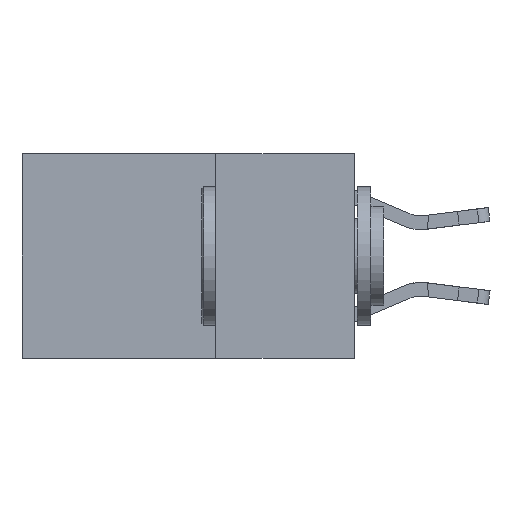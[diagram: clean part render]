
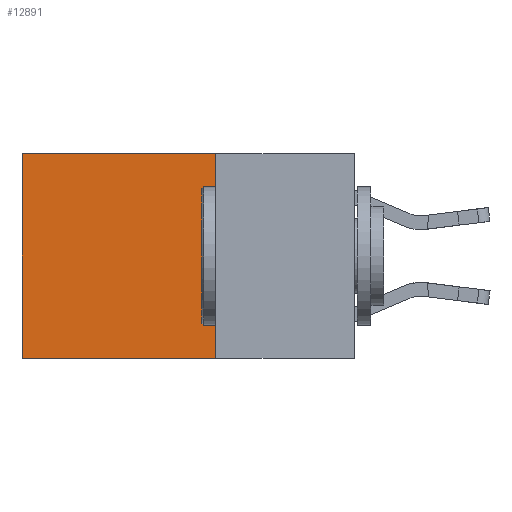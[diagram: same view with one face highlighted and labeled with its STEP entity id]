
A CAD part, left-side view. The second image highlights one B-rep face of the part: STEP entity #12891.
In plain terms, the highlighted planar face has unit normal (-1, 0, 0).
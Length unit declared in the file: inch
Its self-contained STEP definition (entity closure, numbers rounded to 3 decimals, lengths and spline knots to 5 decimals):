
#623 = AXIS2_PLACEMENT_3D ( 'NONE', #16962, #15904, #2747 ) ;
#1274 = VERTEX_POINT ( 'NONE', #6237 ) ;
#1574 = CARTESIAN_POINT ( 'NONE',  ( 0.2625, 0.25, 0. ) ) ;
#2537 = LINE ( 'NONE', #6964, #4032 ) ;
#2646 = PLANE ( 'NONE',  #623 ) ;
#2747 = DIRECTION ( 'NONE',  ( 0., 0., -1. ) ) ;
#2769 = ORIENTED_EDGE ( 'NONE', *, *, #17958, .F. ) ;
#3124 = VERTEX_POINT ( 'NONE', #14053 ) ;
#3986 = FACE_OUTER_BOUND ( 'NONE', #12010, .T. ) ;
#4032 = VECTOR ( 'NONE', #13962, 39.37008 ) ;
#6237 = CARTESIAN_POINT ( 'NONE',  ( 0.2625, 0.6, -0.37 ) ) ;
#6335 = EDGE_CURVE ( 'NONE', #3124, #1274, #2537, .T. ) ;
#6521 = DIRECTION ( 'NONE',  ( 0., 0., -1. ) ) ;
#6964 = CARTESIAN_POINT ( 'NONE',  ( 0.2625, 0.6, 0. ) ) ;
#7256 = DIRECTION ( 'NONE',  ( 0., 1., 0. ) ) ;
#7347 = LINE ( 'NONE', #1574, #14202 ) ;
#8284 = ORIENTED_EDGE ( 'NONE', *, *, #6335, .T. ) ;
#8939 = EDGE_CURVE ( 'NONE', #15135, #14184, #18432, .T. ) ;
#9906 = CARTESIAN_POINT ( 'NONE',  ( 0.2625, 0.25, 0. ) ) ;
#10504 = LINE ( 'NONE', #13473, #16674 ) ;
#11165 = VECTOR ( 'NONE', #6521, 39.37008 ) ;
#12010 = EDGE_LOOP ( 'NONE', ( #8284, #2769, #17851, #18306 ) ) ;
#12643 = CARTESIAN_POINT ( 'NONE',  ( 0.2625, 0.25, 0. ) ) ;
#12649 = CARTESIAN_POINT ( 'NONE',  ( 0.2625, 0.25, -0.37 ) ) ;
#12891 = ADVANCED_FACE ( 'NONE', ( #3986 ), #2646, .F. ) ;
#13473 = CARTESIAN_POINT ( 'NONE',  ( 0.2625, 0.25, -0.37 ) ) ;
#13962 = DIRECTION ( 'NONE',  ( 0., 0., -1. ) ) ;
#14053 = CARTESIAN_POINT ( 'NONE',  ( 0.2625, 0.6, 0. ) ) ;
#14184 = VERTEX_POINT ( 'NONE', #12649 ) ;
#14202 = VECTOR ( 'NONE', #16278, 39.37008 ) ;
#15135 = VERTEX_POINT ( 'NONE', #9906 ) ;
#15904 = DIRECTION ( 'NONE',  ( 1., 0., 0. ) ) ;
#16278 = DIRECTION ( 'NONE',  ( 0., 1., 0. ) ) ;
#16674 = VECTOR ( 'NONE', #7256, 39.37008 ) ;
#16962 = CARTESIAN_POINT ( 'NONE',  ( 0.2625, 0.25, 0. ) ) ;
#17851 = ORIENTED_EDGE ( 'NONE', *, *, #8939, .F. ) ;
#17958 = EDGE_CURVE ( 'NONE', #14184, #1274, #10504, .T. ) ;
#18008 = EDGE_CURVE ( 'NONE', #15135, #3124, #7347, .T. ) ;
#18306 = ORIENTED_EDGE ( 'NONE', *, *, #18008, .T. ) ;
#18432 = LINE ( 'NONE', #12643, #11165 ) ;
